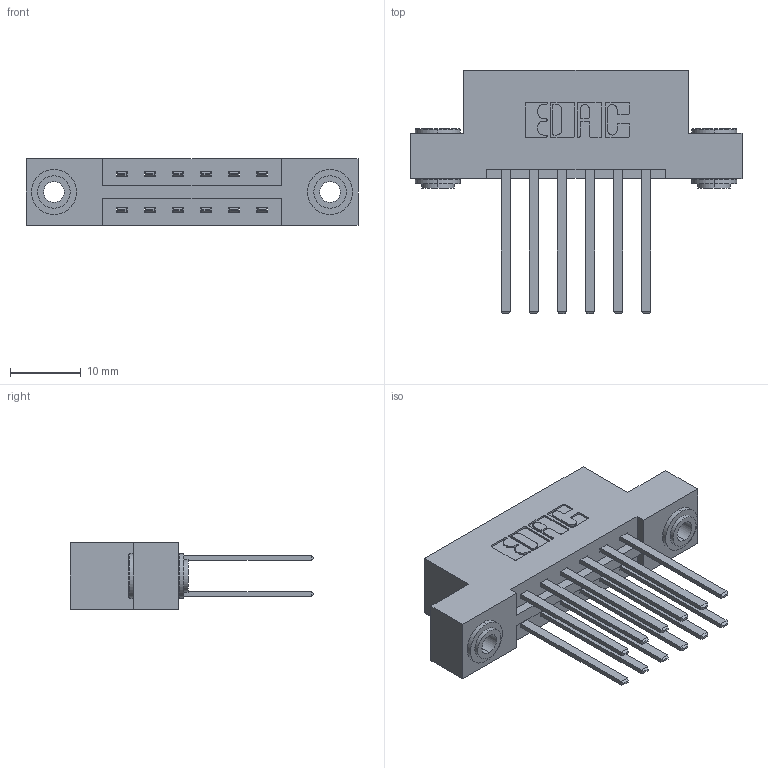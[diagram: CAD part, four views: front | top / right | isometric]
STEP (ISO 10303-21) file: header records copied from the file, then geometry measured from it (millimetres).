
FILE_DESCRIPTION (( 'STEP AP203' ), '1' );
FILE_NAME ('387-012-544-203.STEP', '2018-09-10T11:58:38', ( '' ), ( '' ), 'SwSTEP 2.0', 'SolidWorks 2016', '' );
FILE_SCHEMA (( 'CONFIG_CONTROL_DESIGN' ));
Length unit declared in the file: inch
Products named in the file (4): 345-250-002_345-250-002-102; 387-012-544-203; 337 Part_Flush Mounting Lugs - 0.156 Dia-TH; 345-292-001_345-293-144
Assembly tree (15 placements, depth 2):
  387-012-544-203
    337 Part_Flush Mounting Lugs - 0.156 Dia-TH
    345-292-001_345-293-144  x12
    345-250-002_345-250-002-102  x2
Bounding box: 46.79 x 34.3 x 9.4 mm (x, y, z)
Volume: 4639.2 mm3; surface area: 5668.8 mm2
Topology: 15 solids, 15 shells, 728 faces, 2103 edges, 1382 vertices
Faces by surface type: plane 488, cylinder 232, cone 8
Entity records: 9774 total; most frequent: CARTESIAN_POINT 1649, ORIENTED_EDGE 1578, DIRECTION 1499, EDGE_CURVE 789, VECTOR 641, LINE 641, VERTEX_POINT 522, AXIS2_PLACEMENT_3D 429
